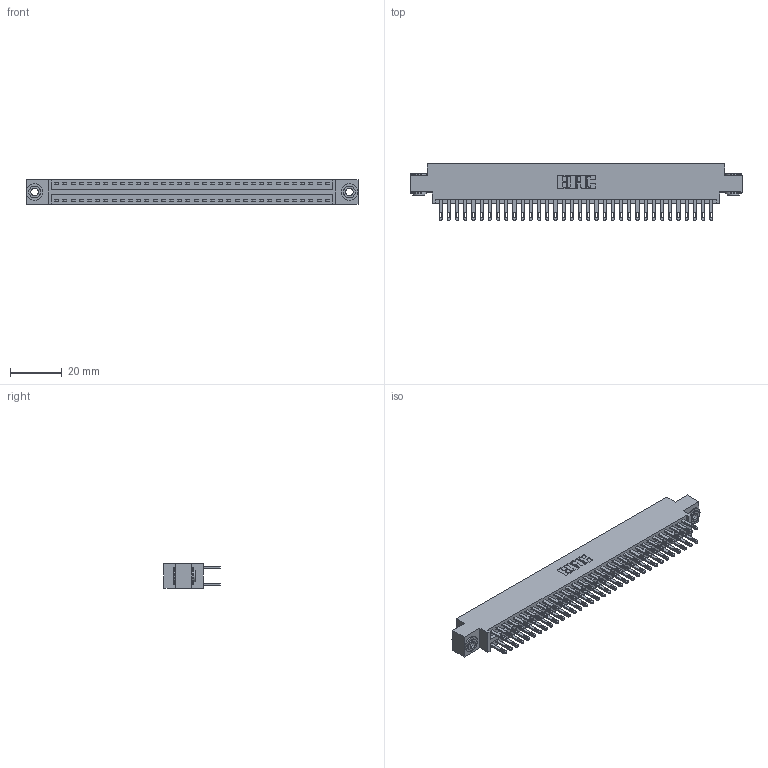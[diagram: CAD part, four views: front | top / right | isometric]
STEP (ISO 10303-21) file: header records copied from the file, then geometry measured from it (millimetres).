
FILE_DESCRIPTION (( 'STEP AP203' ), '1' );
FILE_NAME ('896-068-500-803.STEP', '2021-07-28T01:05:38', ( '' ), ( '' ), 'SwSTEP 2.0', 'SolidWorks 2020', '' );
FILE_SCHEMA (( 'CONFIG_CONTROL_DESIGN' ));
Length unit declared in the file: inch
Products named in the file (4): 896-068-500-803; 345-250-002_345-250-002-102; 846 Part_0.170 Offset - 0.156 Dia-TH; 345-292-001_345-293-100
Assembly tree (71 placements, depth 2):
  896-068-500-803
    846 Part_0.170 Offset - 0.156 Dia-TH
    345-292-001_345-293-100  x68
    345-250-002_345-250-002-102  x2
Bounding box: 128.52 x 21.84 x 9.4 mm (x, y, z)
Volume: 12543.1 mm3; surface area: 18221.2 mm2
Topology: 71 solids, 71 shells, 3428 faces, 10413 edges, 6938 vertices
Faces by surface type: plane 2062, cylinder 1358, cone 8
Entity records: 23978 total; most frequent: CARTESIAN_POINT 3939, ORIENTED_EDGE 3866, DIRECTION 3555, EDGE_CURVE 1933, LINE 1637, VECTOR 1637, VERTEX_POINT 1286, AXIS2_PLACEMENT_3D 959
